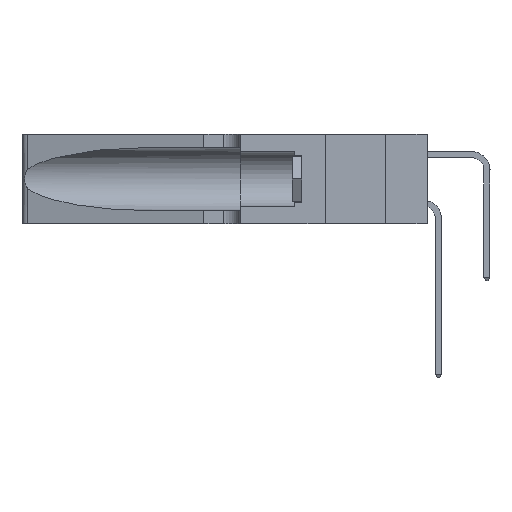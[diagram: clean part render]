
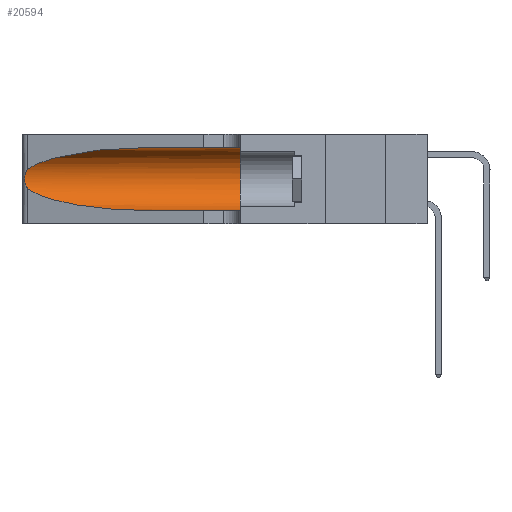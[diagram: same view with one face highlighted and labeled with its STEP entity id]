
A CAD part, left-side view. The second image highlights one B-rep face of the part: STEP entity #20594.
In plain terms, the highlighted cylindrical face has radius 3.308 mm (diameter 6.617 mm), a partial arc.
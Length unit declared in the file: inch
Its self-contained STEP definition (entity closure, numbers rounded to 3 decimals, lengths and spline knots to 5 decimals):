
#119 = EDGE_CURVE ( 'NONE', #25996, #32503, #17427, .T. ) ;
#1259 = DIRECTION ( 'NONE',  ( 0., 0., -1. ) ) ;
#1455 = CARTESIAN_POINT ( 'NONE',  ( 0.25555, 1.22994, 0.2215 ) ) ;
#1598 = AXIS2_PLACEMENT_3D ( 'NONE', #9054, #3652, #23156 ) ;
#1689 = CARTESIAN_POINT ( 'NONE',  ( 0.25854, 1.2359, 0.20912 ) ) ;
#2989 = CARTESIAN_POINT ( 'NONE',  ( 0.18966, 0.96281, 0.05475 ) ) ;
#3094 = ORIENTED_EDGE ( 'NONE', *, *, #31588, .F. ) ;
#3494 = LINE ( 'NONE', #18679, #16169 ) ;
#3652 = DIRECTION ( 'NONE',  ( 0., 1., 0. ) ) ;
#4043 = AXIS2_PLACEMENT_3D ( 'NONE', #6336, #31544, #1259 ) ;
#4606 = VERTEX_POINT ( 'NONE', #17780 ) ;
#5573 = CARTESIAN_POINT ( 'NONE',  ( 0.2373, 1.15595, 0.08982 ) ) ;
#6336 = CARTESIAN_POINT ( 'NONE',  ( 0.1305, 1.61858, 0.185 ) ) ;
#6459 = CARTESIAN_POINT ( 'NONE',  ( 0.1305, 0.35, 0.05475 ) ) ;
#7367 = CARTESIAN_POINT ( 'NONE',  ( 0.26018, 1.23835, 0.19895 ) ) ;
#8399 = ORIENTED_EDGE ( 'NONE', *, *, #16204, .F. ) ;
#9054 = CARTESIAN_POINT ( 'NONE',  ( 0.1305, 0.35, 0.185 ) ) ;
#9258 = DIRECTION ( 'NONE',  ( 0., -1., 0. ) ) ;
#10131 = ORIENTED_EDGE ( 'NONE', *, *, #10886, .T. ) ;
#10320 = CARTESIAN_POINT ( 'NONE',  ( 0.26075, 1.23896, 0.178 ) ) ;
#10450 = CARTESIAN_POINT ( 'NONE',  ( 0.25487, 1.22718, 0.14631 ) ) ;
#10886 = EDGE_CURVE ( 'NONE', #32503, #23934, #3494, .T. ) ;
#12068 = CARTESIAN_POINT ( 'NONE',  ( 0.25487, 1.22718, 0.22369 ) ) ;
#12079 = CARTESIAN_POINT ( 'NONE',  ( 0.25487, 1.22718, 0.22369 ) ) ;
#12440 = CARTESIAN_POINT ( 'NONE',  ( 0.2373, 1.15595, 0.28018 ) ) ;
#12671 = VECTOR ( 'NONE', #9258, 39.37008 ) ;
#13379 = ORIENTED_EDGE ( 'NONE', *, *, #27920, .T. ) ;
#16169 = VECTOR ( 'NONE', #35496, 39.37008 ) ;
#16204 = EDGE_CURVE ( 'NONE', #28140, #23934, #22174, .T. ) ;
#16580 = CARTESIAN_POINT ( 'NONE',  ( 0.25487, 1.22718, 0.14631 ) ) ;
#17223 = ORIENTED_EDGE ( 'NONE', *, *, #23538, .T. ) ;
#17427 =( BOUNDED_CURVE ( )  B_SPLINE_CURVE ( 3, ( #16580, #5573, #2989, #30652 ),
 .UNSPECIFIED., .F., .T. ) 
 B_SPLINE_CURVE_WITH_KNOTS ( ( 4, 4 ),
 ( 3.44316, 4.71239 ),
 .UNSPECIFIED. ) 
 CURVE ( )  GEOMETRIC_REPRESENTATION_ITEM ( )  RATIONAL_B_SPLINE_CURVE ( ( 1., 0.87, 0.87, 1. ) ) 
 REPRESENTATION_ITEM ( '' )  );
#17780 = CARTESIAN_POINT ( 'NONE',  ( 0.1305, 0.72297, 0.31525 ) ) ;
#18337 = VERTEX_POINT ( 'NONE', #27948 ) ;
#18648 = CARTESIAN_POINT ( 'NONE',  ( 0.1305, 0.35, 0.31525 ) ) ;
#18679 = CARTESIAN_POINT ( 'NONE',  ( 0.1305, 1.61858, 0.05475 ) ) ;
#19129 = CARTESIAN_POINT ( 'NONE',  ( 0.25856, 1.23593, 0.16098 ) ) ;
#19305 = CARTESIAN_POINT ( 'NONE',  ( 0.25487, 1.22718, 0.14631 ) ) ;
#20439 = ORIENTED_EDGE ( 'NONE', *, *, #119, .T. ) ;
#20594 = ADVANCED_FACE ( 'NONE', ( #21941 ), #35499, .F. ) ;
#20775 = B_SPLINE_CURVE_WITH_KNOTS ( 'NONE', 3,
 ( #12068, #1455, #26602, #23908, #1689, #7367, #21449, #10320, #27450, #19129, #24869, #29875, #21580, #10450 ),
 .UNSPECIFIED., .F., .F.,
 ( 4, 2, 2, 2, 2, 2, 4 ),
 ( 0., 0.00027, 0.00053, 0.00107, 0.0016, 0.00187, 0.00214 ),
 .UNSPECIFIED. ) ;
#21449 = CARTESIAN_POINT ( 'NONE',  ( 0.26075, 1.23896, 0.19203 ) ) ;
#21580 = CARTESIAN_POINT ( 'NONE',  ( 0.25555, 1.22993, 0.14849 ) ) ;
#21941 = FACE_OUTER_BOUND ( 'NONE', #24158, .T. ) ;
#22174 = CIRCLE ( 'NONE', #1598, 0.13025 ) ;
#23156 = DIRECTION ( 'NONE',  ( 0., 0., 1. ) ) ;
#23538 = EDGE_CURVE ( 'NONE', #18337, #25996, #20775, .T. ) ;
#23908 = CARTESIAN_POINT ( 'NONE',  ( 0.25787, 1.23484, 0.2124 ) ) ;
#23934 = VERTEX_POINT ( 'NONE', #6459 ) ;
#24158 = EDGE_LOOP ( 'NONE', ( #13379, #17223, #20439, #10131, #8399, #3094 ) ) ;
#24869 = CARTESIAN_POINT ( 'NONE',  ( 0.25789, 1.23486, 0.15765 ) ) ;
#25996 = VERTEX_POINT ( 'NONE', #19305 ) ;
#26268 = CARTESIAN_POINT ( 'NONE',  ( 0.1305, 1.61858, 0.31525 ) ) ;
#26383 = CARTESIAN_POINT ( 'NONE',  ( 0.1305, 0.72297, 0.31525 ) ) ;
#26602 = CARTESIAN_POINT ( 'NONE',  ( 0.25639, 1.23184, 0.21858 ) ) ;
#27450 = CARTESIAN_POINT ( 'NONE',  ( 0.26017, 1.23833, 0.17102 ) ) ;
#27920 = EDGE_CURVE ( 'NONE', #4606, #18337, #30394, .T. ) ;
#27948 = CARTESIAN_POINT ( 'NONE',  ( 0.25487, 1.22718, 0.22369 ) ) ;
#27959 = LINE ( 'NONE', #26268, #12671 ) ;
#28140 = VERTEX_POINT ( 'NONE', #18648 ) ;
#29875 = CARTESIAN_POINT ( 'NONE',  ( 0.25639, 1.23186, 0.15144 ) ) ;
#30394 =( BOUNDED_CURVE ( )  B_SPLINE_CURVE ( 3, ( #26383, #31748, #12440, #12079 ),
 .UNSPECIFIED., .F., .F. ) 
 B_SPLINE_CURVE_WITH_KNOTS ( ( 4, 4 ),
 ( 1.5708, 2.84003 ),
 .UNSPECIFIED. ) 
 CURVE ( )  GEOMETRIC_REPRESENTATION_ITEM ( )  RATIONAL_B_SPLINE_CURVE ( ( 1., 0.87, 0.87, 1. ) ) 
 REPRESENTATION_ITEM ( '' )  );
#30652 = CARTESIAN_POINT ( 'NONE',  ( 0.1305, 0.72297, 0.05475 ) ) ;
#31544 = DIRECTION ( 'NONE',  ( 0., -1., 0. ) ) ;
#31588 = EDGE_CURVE ( 'NONE', #4606, #28140, #27959, .T. ) ;
#31748 = CARTESIAN_POINT ( 'NONE',  ( 0.18966, 0.96281, 0.31525 ) ) ;
#32503 = VERTEX_POINT ( 'NONE', #35953 ) ;
#35496 = DIRECTION ( 'NONE',  ( 0., -1., 0. ) ) ;
#35499 = CYLINDRICAL_SURFACE ( 'NONE', #4043, 0.13025 ) ;
#35953 = CARTESIAN_POINT ( 'NONE',  ( 0.1305, 0.72297, 0.05475 ) ) ;
